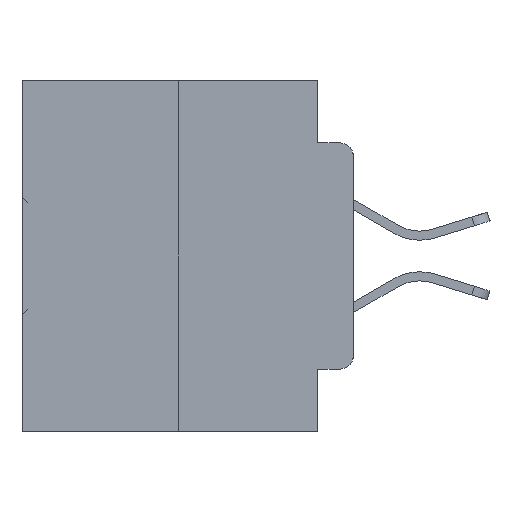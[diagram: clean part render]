
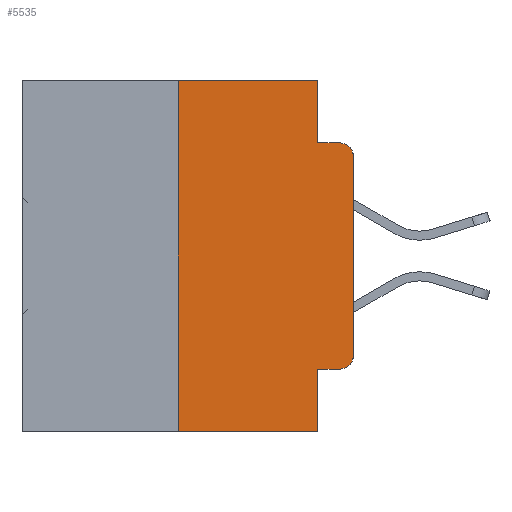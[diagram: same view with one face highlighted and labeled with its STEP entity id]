
A CAD part, left-side view. The second image highlights one B-rep face of the part: STEP entity #5535.
In plain terms, the highlighted planar face has unit normal (-1, 0, 0).
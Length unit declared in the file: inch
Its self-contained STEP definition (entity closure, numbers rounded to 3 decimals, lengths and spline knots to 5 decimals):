
#138 = DIRECTION ( 'NONE',  ( 0., -1., 0. ) ) ;
#150 = CARTESIAN_POINT ( 'NONE',  ( 0., 0.051, 0. ) ) ;
#1872 = CARTESIAN_POINT ( 'NONE',  ( 0., 0.051, -0.5 ) ) ;
#1931 = ORIENTED_EDGE ( 'NONE', *, *, #17983, .T. ) ;
#2048 = ORIENTED_EDGE ( 'NONE', *, *, #19361, .F. ) ;
#2887 = AXIS2_PLACEMENT_3D ( 'NONE', #31124, #6229, #17332 ) ;
#2896 = CARTESIAN_POINT ( 'NONE',  ( 0., 0.473, 0. ) ) ;
#3094 = DIRECTION ( 'NONE',  ( -1., 0., 0. ) ) ;
#3438 = ORIENTED_EDGE ( 'NONE', *, *, #9262, .F. ) ;
#3691 = CARTESIAN_POINT ( 'NONE',  ( 0., 0.25, -0.5 ) ) ;
#4199 = LINE ( 'NONE', #150, #7456 ) ;
#5309 = VECTOR ( 'NONE', #23851, 39.37008 ) ;
#5535 = ADVANCED_FACE ( 'NONE', ( #31011 ), #13637, .F. ) ;
#5819 = CIRCLE ( 'NONE', #11624, 0.02 ) ;
#5825 = CARTESIAN_POINT ( 'NONE',  ( 0., 0.02, -0.3915 ) ) ;
#6229 = DIRECTION ( 'NONE',  ( -1., 0., 0. ) ) ;
#6720 = ORIENTED_EDGE ( 'NONE', *, *, #9303, .F. ) ;
#6821 = CARTESIAN_POINT ( 'NONE',  ( 0., 0.051, 0. ) ) ;
#6990 = VERTEX_POINT ( 'NONE', #21959 ) ;
#7456 = VECTOR ( 'NONE', #25083, 39.37008 ) ;
#8714 = DIRECTION ( 'NONE',  ( 0., -1., 0. ) ) ;
#9262 = EDGE_CURVE ( 'NONE', #19561, #33162, #27789, .T. ) ;
#9303 = EDGE_CURVE ( 'NONE', #20630, #19561, #11984, .T. ) ;
#9819 = VECTOR ( 'NONE', #34198, 39.37008 ) ;
#9832 = LINE ( 'NONE', #15484, #22515 ) ;
#9881 = CARTESIAN_POINT ( 'NONE',  ( 0., 0.051, -0.4115 ) ) ;
#10260 = ORIENTED_EDGE ( 'NONE', *, *, #34998, .F. ) ;
#10721 = CARTESIAN_POINT ( 'NONE',  ( 0., 0.051, -0.0885 ) ) ;
#11043 = CARTESIAN_POINT ( 'NONE',  ( 0., 0., -0.1085 ) ) ;
#11624 = AXIS2_PLACEMENT_3D ( 'NONE', #5825, #3094, #14190 ) ;
#11703 = ORIENTED_EDGE ( 'NONE', *, *, #33910, .T. ) ;
#11840 = CARTESIAN_POINT ( 'NONE',  ( 0., 0.473, -0.5 ) ) ;
#11984 = LINE ( 'NONE', #25781, #23503 ) ;
#12062 = VECTOR ( 'NONE', #8714, 39.37008 ) ;
#12068 = EDGE_CURVE ( 'NONE', #31966, #12570, #9832, .T. ) ;
#12158 = EDGE_CURVE ( 'NONE', #21338, #25728, #14012, .T. ) ;
#12570 = VERTEX_POINT ( 'NONE', #11043 ) ;
#12906 = VERTEX_POINT ( 'NONE', #1872 ) ;
#13358 = CARTESIAN_POINT ( 'NONE',  ( 0., 0.051, -0.4115 ) ) ;
#13625 = CARTESIAN_POINT ( 'NONE',  ( 0., 0.051, -0.0885 ) ) ;
#13637 = PLANE ( 'NONE',  #26241 ) ;
#14012 = LINE ( 'NONE', #10721, #12062 ) ;
#14190 = DIRECTION ( 'NONE',  ( 0., 0., -1. ) ) ;
#15359 = VECTOR ( 'NONE', #138, 39.37008 ) ;
#15484 = CARTESIAN_POINT ( 'NONE',  ( 0., 0., 0. ) ) ;
#15497 = CARTESIAN_POINT ( 'NONE',  ( 0., 0.02, -0.0885 ) ) ;
#15501 = LINE ( 'NONE', #24030, #5309 ) ;
#15556 = VERTEX_POINT ( 'NONE', #9881 ) ;
#16330 = EDGE_CURVE ( 'NONE', #6990, #31966, #5819, .T. ) ;
#17332 = DIRECTION ( 'NONE',  ( 0., 0., -1. ) ) ;
#17578 = DIRECTION ( 'NONE',  ( 1., 0., 0. ) ) ;
#17890 = ORIENTED_EDGE ( 'NONE', *, *, #12158, .F. ) ;
#17983 = EDGE_CURVE ( 'NONE', #12570, #25728, #33658, .T. ) ;
#18849 = ORIENTED_EDGE ( 'NONE', *, *, #18992, .T. ) ;
#18992 = EDGE_CURVE ( 'NONE', #15556, #6990, #27149, .T. ) ;
#19361 = EDGE_CURVE ( 'NONE', #33162, #21338, #15501, .T. ) ;
#19561 = VERTEX_POINT ( 'NONE', #28182 ) ;
#20136 = DIRECTION ( 'NONE',  ( 0., 0., -1. ) ) ;
#20630 = VERTEX_POINT ( 'NONE', #3691 ) ;
#21338 = VERTEX_POINT ( 'NONE', #13625 ) ;
#21959 = CARTESIAN_POINT ( 'NONE',  ( 0., 0.02, -0.4115 ) ) ;
#22054 = EDGE_LOOP ( 'NONE', ( #27349, #1931, #17890, #2048, #3438, #6720, #11703, #10260, #18849, #30324 ) ) ;
#22515 = VECTOR ( 'NONE', #26553, 39.37008 ) ;
#23503 = VECTOR ( 'NONE', #34154, 39.37008 ) ;
#23851 = DIRECTION ( 'NONE',  ( 0., 0., -1. ) ) ;
#23892 = DIRECTION ( 'NONE',  ( 0., -1., 0. ) ) ;
#24030 = CARTESIAN_POINT ( 'NONE',  ( 0., 0.051, 0. ) ) ;
#25083 = DIRECTION ( 'NONE',  ( 0., 0., -1. ) ) ;
#25385 = CARTESIAN_POINT ( 'NONE',  ( 0., 0.473, 0. ) ) ;
#25728 = VERTEX_POINT ( 'NONE', #15497 ) ;
#25781 = CARTESIAN_POINT ( 'NONE',  ( 0., 0.25, 0. ) ) ;
#25825 = LINE ( 'NONE', #11840, #9819 ) ;
#26241 = AXIS2_PLACEMENT_3D ( 'NONE', #25385, #17578, #20136 ) ;
#26553 = DIRECTION ( 'NONE',  ( 0., 0., 1. ) ) ;
#27149 = LINE ( 'NONE', #13358, #31967 ) ;
#27349 = ORIENTED_EDGE ( 'NONE', *, *, #12068, .T. ) ;
#27789 = LINE ( 'NONE', #2896, #15359 ) ;
#28182 = CARTESIAN_POINT ( 'NONE',  ( 0., 0.25, 0. ) ) ;
#30324 = ORIENTED_EDGE ( 'NONE', *, *, #16330, .T. ) ;
#31011 = FACE_OUTER_BOUND ( 'NONE', #22054, .T. ) ;
#31124 = CARTESIAN_POINT ( 'NONE',  ( 0., 0.02, -0.1085 ) ) ;
#31966 = VERTEX_POINT ( 'NONE', #32252 ) ;
#31967 = VECTOR ( 'NONE', #23892, 39.37008 ) ;
#32252 = CARTESIAN_POINT ( 'NONE',  ( 0., 0., -0.3915 ) ) ;
#33162 = VERTEX_POINT ( 'NONE', #6821 ) ;
#33658 = CIRCLE ( 'NONE', #2887, 0.02 ) ;
#33910 = EDGE_CURVE ( 'NONE', #20630, #12906, #25825, .T. ) ;
#34154 = DIRECTION ( 'NONE',  ( 0., 0., 1. ) ) ;
#34198 = DIRECTION ( 'NONE',  ( 0., -1., 0. ) ) ;
#34998 = EDGE_CURVE ( 'NONE', #15556, #12906, #4199, .T. ) ;
